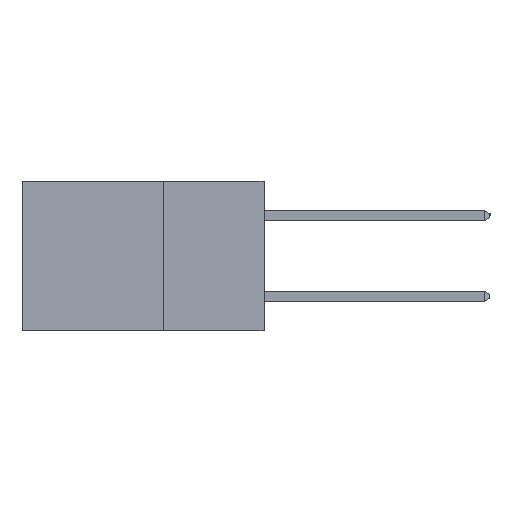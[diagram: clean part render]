
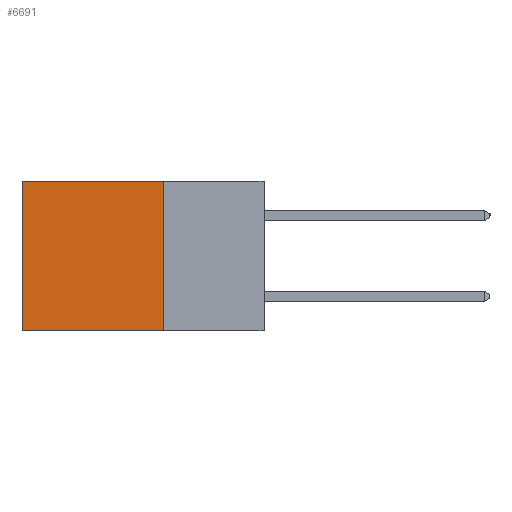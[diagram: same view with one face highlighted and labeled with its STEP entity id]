
A CAD part, left-side view. The second image highlights one B-rep face of the part: STEP entity #6691.
In plain terms, the highlighted planar face has unit normal (-1, 0, 0).
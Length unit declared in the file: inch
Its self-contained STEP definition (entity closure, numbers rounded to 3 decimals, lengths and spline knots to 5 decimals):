
#22 = CARTESIAN_POINT ( 'NONE',  ( 0.2615, 0.25, -0.37 ) ) ;
#478 = DIRECTION ( 'NONE',  ( 0., 0., -1. ) ) ;
#749 = ORIENTED_EDGE ( 'NONE', *, *, #11441, .F. ) ;
#934 = LINE ( 'NONE', #5865, #11867 ) ;
#981 = CARTESIAN_POINT ( 'NONE',  ( 0.2615, 0.6, -0.37 ) ) ;
#1116 = DIRECTION ( 'NONE',  ( 0., 1., 0. ) ) ;
#1275 = EDGE_CURVE ( 'NONE', #9110, #2867, #2151, .T. ) ;
#2151 = LINE ( 'NONE', #5145, #6167 ) ;
#2248 = EDGE_CURVE ( 'NONE', #2867, #9548, #5222, .T. ) ;
#2463 = CARTESIAN_POINT ( 'NONE',  ( 0.2615, 0.25, -0.37 ) ) ;
#2867 = VERTEX_POINT ( 'NONE', #11508 ) ;
#3124 = DIRECTION ( 'NONE',  ( 0., 0., -1. ) ) ;
#3417 = LINE ( 'NONE', #2463, #10515 ) ;
#3539 = DIRECTION ( 'NONE',  ( 0., 0., -1. ) ) ;
#4150 = DIRECTION ( 'NONE',  ( 0., 1., 0. ) ) ;
#5145 = CARTESIAN_POINT ( 'NONE',  ( 0.2615, 0.25, 0. ) ) ;
#5190 = VERTEX_POINT ( 'NONE', #9225 ) ;
#5222 = LINE ( 'NONE', #8145, #9158 ) ;
#5754 = EDGE_LOOP ( 'NONE', ( #7210, #10906, #749, #11594 ) ) ;
#5865 = CARTESIAN_POINT ( 'NONE',  ( 0.2615, 0.25, -0.37 ) ) ;
#6167 = VECTOR ( 'NONE', #4150, 39.37008 ) ;
#6691 = ADVANCED_FACE ( 'NONE', ( #11606 ), #7864, .F. ) ;
#6755 = EDGE_CURVE ( 'NONE', #5190, #9548, #934, .T. ) ;
#6954 = AXIS2_PLACEMENT_3D ( 'NONE', #22, #11666, #3124 ) ;
#7210 = ORIENTED_EDGE ( 'NONE', *, *, #2248, .T. ) ;
#7864 = PLANE ( 'NONE',  #6954 ) ;
#8145 = CARTESIAN_POINT ( 'NONE',  ( 0.2615, 0.6, -0.37 ) ) ;
#9110 = VERTEX_POINT ( 'NONE', #10974 ) ;
#9158 = VECTOR ( 'NONE', #478, 39.37008 ) ;
#9225 = CARTESIAN_POINT ( 'NONE',  ( 0.2615, 0.25, -0.37 ) ) ;
#9548 = VERTEX_POINT ( 'NONE', #981 ) ;
#10515 = VECTOR ( 'NONE', #3539, 39.37008 ) ;
#10906 = ORIENTED_EDGE ( 'NONE', *, *, #6755, .F. ) ;
#10974 = CARTESIAN_POINT ( 'NONE',  ( 0.2615, 0.25, 0. ) ) ;
#11441 = EDGE_CURVE ( 'NONE', #9110, #5190, #3417, .T. ) ;
#11508 = CARTESIAN_POINT ( 'NONE',  ( 0.2615, 0.6, 0. ) ) ;
#11594 = ORIENTED_EDGE ( 'NONE', *, *, #1275, .T. ) ;
#11606 = FACE_OUTER_BOUND ( 'NONE', #5754, .T. ) ;
#11666 = DIRECTION ( 'NONE',  ( 1., 0., 0. ) ) ;
#11867 = VECTOR ( 'NONE', #1116, 39.37008 ) ;
